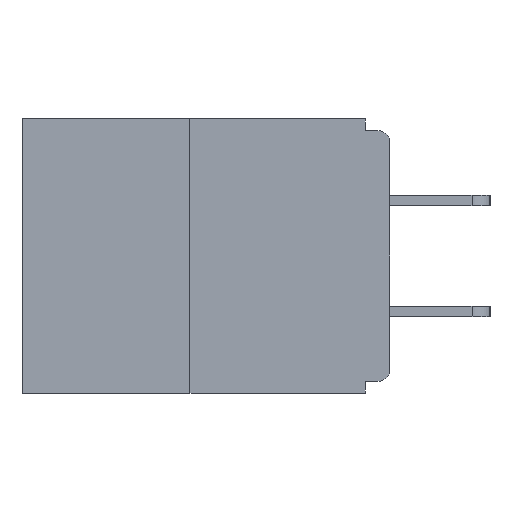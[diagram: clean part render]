
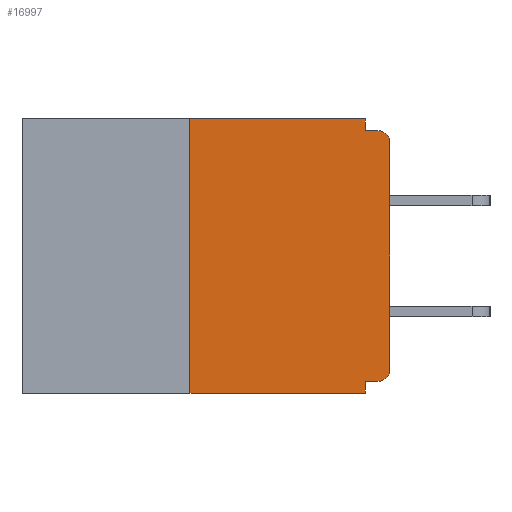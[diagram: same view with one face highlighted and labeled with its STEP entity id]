
A CAD part, left-side view. The second image highlights one B-rep face of the part: STEP entity #16997.
In plain terms, the highlighted planar face has unit normal (-1, 0, 0).
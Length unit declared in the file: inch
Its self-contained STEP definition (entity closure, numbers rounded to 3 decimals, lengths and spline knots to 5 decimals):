
#686 = EDGE_CURVE ( 'NONE', #1141, #16180, #24019, .T. ) ;
#951 = VERTEX_POINT ( 'NONE', #2774 ) ;
#1054 = VECTOR ( 'NONE', #10749, 39.37008 ) ;
#1141 = VERTEX_POINT ( 'NONE', #11119 ) ;
#1311 = ORIENTED_EDGE ( 'NONE', *, *, #10447, .F. ) ;
#1335 = VECTOR ( 'NONE', #20710, 39.37008 ) ;
#2246 = CARTESIAN_POINT ( 'NONE',  ( 0., 0.015, -0.015 ) ) ;
#2248 = CARTESIAN_POINT ( 'NONE',  ( 0., 0.015, -0.313 ) ) ;
#2728 = DIRECTION ( 'NONE',  ( 0., -1., 0. ) ) ;
#2774 = CARTESIAN_POINT ( 'NONE',  ( 0., 0.25, -0.343 ) ) ;
#2969 = VECTOR ( 'NONE', #2728, 39.37008 ) ;
#3544 = LINE ( 'NONE', #9164, #24202 ) ;
#3743 = CARTESIAN_POINT ( 'NONE',  ( 0., 0.031, 0. ) ) ;
#4234 = DIRECTION ( 'NONE',  ( -1., 0., 0. ) ) ;
#4482 = EDGE_CURVE ( 'NONE', #19128, #7103, #10764, .T. ) ;
#4652 = VECTOR ( 'NONE', #28753, 39.37008 ) ;
#5135 = CARTESIAN_POINT ( 'NONE',  ( 0., 0.46, 0. ) ) ;
#5590 = AXIS2_PLACEMENT_3D ( 'NONE', #29753, #9627, #11780 ) ;
#7103 = VERTEX_POINT ( 'NONE', #13727 ) ;
#7492 = VERTEX_POINT ( 'NONE', #19933 ) ;
#7532 = EDGE_CURVE ( 'NONE', #951, #12182, #28110, .T. ) ;
#7932 = CARTESIAN_POINT ( 'NONE',  ( 0., 0., 0. ) ) ;
#8121 = ORIENTED_EDGE ( 'NONE', *, *, #13225, .T. ) ;
#8298 = LINE ( 'NONE', #7932, #4652 ) ;
#9164 = CARTESIAN_POINT ( 'NONE',  ( 0., 0.46, -0.343 ) ) ;
#9627 = DIRECTION ( 'NONE',  ( 1., 0., 0. ) ) ;
#9726 = ORIENTED_EDGE ( 'NONE', *, *, #16010, .F. ) ;
#9978 = ORIENTED_EDGE ( 'NONE', *, *, #19964, .F. ) ;
#10200 = CARTESIAN_POINT ( 'NONE',  ( 0., 0.015, -0.328 ) ) ;
#10284 = CARTESIAN_POINT ( 'NONE',  ( 0., 0., -0.328 ) ) ;
#10447 = EDGE_CURVE ( 'NONE', #12182, #7492, #28286, .T. ) ;
#10749 = DIRECTION ( 'NONE',  ( 0., 0., -1. ) ) ;
#10764 = CIRCLE ( 'NONE', #20372, 0.015 ) ;
#10800 = ORIENTED_EDGE ( 'NONE', *, *, #7532, .F. ) ;
#11119 = CARTESIAN_POINT ( 'NONE',  ( 0., 0.031, -0.015 ) ) ;
#11182 = DIRECTION ( 'NONE',  ( 0., 0., -1. ) ) ;
#11652 = EDGE_CURVE ( 'NONE', #7492, #1141, #18782, .T. ) ;
#11780 = DIRECTION ( 'NONE',  ( 0., 0., -1. ) ) ;
#12182 = VERTEX_POINT ( 'NONE', #25617 ) ;
#12485 = EDGE_CURVE ( 'NONE', #23147, #16180, #23475, .T. ) ;
#12804 = VERTEX_POINT ( 'NONE', #24377 ) ;
#12960 = EDGE_LOOP ( 'NONE', ( #1311, #10800, #26374, #9726, #9978, #24963, #8121, #13783, #22819, #26140 ) ) ;
#13081 = CARTESIAN_POINT ( 'NONE',  ( 0., 0.031, -0.343 ) ) ;
#13225 = EDGE_CURVE ( 'NONE', #7103, #23147, #8298, .T. ) ;
#13727 = CARTESIAN_POINT ( 'NONE',  ( 0., 0., -0.313 ) ) ;
#13783 = ORIENTED_EDGE ( 'NONE', *, *, #12485, .T. ) ;
#13798 = EDGE_CURVE ( 'NONE', #951, #14225, #3544, .T. ) ;
#14133 = CARTESIAN_POINT ( 'NONE',  ( 0., 0.25, 0. ) ) ;
#14225 = VERTEX_POINT ( 'NONE', #18950 ) ;
#15408 = DIRECTION ( 'NONE',  ( 0., 0., -1. ) ) ;
#15842 = DIRECTION ( 'NONE',  ( 0., -1., 0. ) ) ;
#16010 = EDGE_CURVE ( 'NONE', #12804, #14225, #29104, .T. ) ;
#16180 = VERTEX_POINT ( 'NONE', #2246 ) ;
#16311 = LINE ( 'NONE', #10284, #21034 ) ;
#16997 = ADVANCED_FACE ( 'NONE', ( #28652 ), #18836, .F. ) ;
#17161 = DIRECTION ( 'NONE',  ( 0., 1., 0. ) ) ;
#17546 = VECTOR ( 'NONE', #15408, 39.37008 ) ;
#18102 = CARTESIAN_POINT ( 'NONE',  ( 0., 0.015, -0.03 ) ) ;
#18782 = LINE ( 'NONE', #3743, #1054 ) ;
#18836 = PLANE ( 'NONE',  #5590 ) ;
#18950 = CARTESIAN_POINT ( 'NONE',  ( 0., 0.031, -0.343 ) ) ;
#19128 = VERTEX_POINT ( 'NONE', #10200 ) ;
#19933 = CARTESIAN_POINT ( 'NONE',  ( 0., 0.031, 0. ) ) ;
#19964 = EDGE_CURVE ( 'NONE', #19128, #12804, #16311, .T. ) ;
#19994 = CARTESIAN_POINT ( 'NONE',  ( 0., 0., -0.015 ) ) ;
#20372 = AXIS2_PLACEMENT_3D ( 'NONE', #2248, #27504, #11182 ) ;
#20427 = DIRECTION ( 'NONE',  ( 0., 0., -1. ) ) ;
#20464 = AXIS2_PLACEMENT_3D ( 'NONE', #18102, #4234, #20427 ) ;
#20710 = DIRECTION ( 'NONE',  ( 0., 0., 1. ) ) ;
#21034 = VECTOR ( 'NONE', #17161, 39.37008 ) ;
#21179 = CARTESIAN_POINT ( 'NONE',  ( 0., 0., -0.03 ) ) ;
#22819 = ORIENTED_EDGE ( 'NONE', *, *, #686, .F. ) ;
#23147 = VERTEX_POINT ( 'NONE', #21179 ) ;
#23286 = VECTOR ( 'NONE', #24154, 39.37008 ) ;
#23475 = CIRCLE ( 'NONE', #20464, 0.015 ) ;
#24019 = LINE ( 'NONE', #19994, #23286 ) ;
#24154 = DIRECTION ( 'NONE',  ( 0., -1., 0. ) ) ;
#24202 = VECTOR ( 'NONE', #15842, 39.37008 ) ;
#24377 = CARTESIAN_POINT ( 'NONE',  ( 0., 0.031, -0.328 ) ) ;
#24963 = ORIENTED_EDGE ( 'NONE', *, *, #4482, .T. ) ;
#25617 = CARTESIAN_POINT ( 'NONE',  ( 0., 0.25, 0. ) ) ;
#26140 = ORIENTED_EDGE ( 'NONE', *, *, #11652, .F. ) ;
#26374 = ORIENTED_EDGE ( 'NONE', *, *, #13798, .T. ) ;
#27504 = DIRECTION ( 'NONE',  ( -1., 0., 0. ) ) ;
#28110 = LINE ( 'NONE', #14133, #1335 ) ;
#28286 = LINE ( 'NONE', #5135, #2969 ) ;
#28652 = FACE_OUTER_BOUND ( 'NONE', #12960, .T. ) ;
#28753 = DIRECTION ( 'NONE',  ( 0., 0., 1. ) ) ;
#29104 = LINE ( 'NONE', #13081, #17546 ) ;
#29753 = CARTESIAN_POINT ( 'NONE',  ( 0., 0.46, 0. ) ) ;
